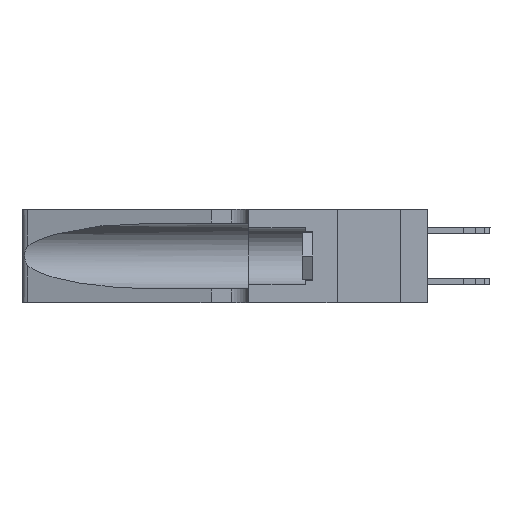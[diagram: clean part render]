
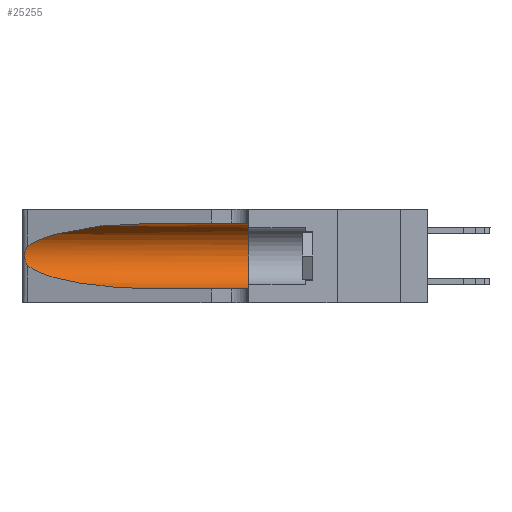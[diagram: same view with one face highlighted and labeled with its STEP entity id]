
A CAD part, left-side view. The second image highlights one B-rep face of the part: STEP entity #25255.
In plain terms, the highlighted cylindrical face has radius 3.308 mm (diameter 6.617 mm), a partial arc.
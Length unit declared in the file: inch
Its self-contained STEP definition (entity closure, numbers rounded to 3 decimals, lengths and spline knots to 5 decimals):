
#773 = DIRECTION ( 'NONE',  ( 0., 0., 1. ) ) ;
#2252 = CARTESIAN_POINT ( 'NONE',  ( 0.1305, 0.72297, 0.31525 ) ) ;
#2629 = LINE ( 'NONE', #6102, #7600 ) ;
#2681 = B_SPLINE_CURVE_WITH_KNOTS ( 'NONE', 3,
 ( #25876, #13319, #20587, #30576, #18399, #15840, #3589, #23060, #10579, #8186, #25547, #28333, #16072, #28000 ),
 .UNSPECIFIED., .F., .F.,
 ( 4, 2, 2, 2, 2, 2, 4 ),
 ( 0., 0.00027, 0.00053, 0.00107, 0.0016, 0.00187, 0.00214 ),
 .UNSPECIFIED. ) ;
#3499 = CARTESIAN_POINT ( 'NONE',  ( 0.1305, 0.35, 0.185 ) ) ;
#3589 = CARTESIAN_POINT ( 'NONE',  ( 0.26075, 1.23896, 0.19203 ) ) ;
#4714 = VERTEX_POINT ( 'NONE', #6596 ) ;
#6102 = CARTESIAN_POINT ( 'NONE',  ( 0.1305, 1.61858, 0.31525 ) ) ;
#6596 = CARTESIAN_POINT ( 'NONE',  ( 0.1305, 0.35, 0.05475 ) ) ;
#7600 = VECTOR ( 'NONE', #18666, 39.37008 ) ;
#7822 = FACE_OUTER_BOUND ( 'NONE', #11271, .T. ) ;
#8050 = CARTESIAN_POINT ( 'NONE',  ( 0.1305, 1.61858, 0.185 ) ) ;
#8186 = CARTESIAN_POINT ( 'NONE',  ( 0.25856, 1.23593, 0.16098 ) ) ;
#8829 = EDGE_CURVE ( 'NONE', #23982, #14994, #9378, .T. ) ;
#8981 = CARTESIAN_POINT ( 'NONE',  ( 0.25487, 1.22718, 0.22369 ) ) ;
#9378 =( BOUNDED_CURVE ( )  B_SPLINE_CURVE ( 3, ( #2252, #29449, #24314, #26797 ),
 .UNSPECIFIED., .F., .T. ) 
 B_SPLINE_CURVE_WITH_KNOTS ( ( 4, 4 ),
 ( 1.5708, 2.84003 ),
 .UNSPECIFIED. ) 
 CURVE ( )  GEOMETRIC_REPRESENTATION_ITEM ( )  RATIONAL_B_SPLINE_CURVE ( ( 1., 0.87, 0.87, 1. ) ) 
 REPRESENTATION_ITEM ( '' )  );
#10579 = CARTESIAN_POINT ( 'NONE',  ( 0.26017, 1.23833, 0.17102 ) ) ;
#10772 =( BOUNDED_CURVE ( )  B_SPLINE_CURVE ( 3, ( #27943, #15438, #13599, #25811 ),
 .UNSPECIFIED., .F., .T. ) 
 B_SPLINE_CURVE_WITH_KNOTS ( ( 4, 4 ),
 ( 3.44316, 4.71239 ),
 .UNSPECIFIED. ) 
 CURVE ( )  GEOMETRIC_REPRESENTATION_ITEM ( )  RATIONAL_B_SPLINE_CURVE ( ( 1., 0.87, 0.87, 1. ) ) 
 REPRESENTATION_ITEM ( '' )  );
#11271 = EDGE_LOOP ( 'NONE', ( #30564, #14636, #17746, #25614, #18194, #31581 ) ) ;
#11343 = LINE ( 'NONE', #31192, #18331 ) ;
#13159 = EDGE_CURVE ( 'NONE', #23982, #17050, #2629, .T. ) ;
#13319 = CARTESIAN_POINT ( 'NONE',  ( 0.25555, 1.22994, 0.2215 ) ) ;
#13599 = CARTESIAN_POINT ( 'NONE',  ( 0.18966, 0.96281, 0.05475 ) ) ;
#13842 = CARTESIAN_POINT ( 'NONE',  ( 0.25487, 1.22718, 0.14631 ) ) ;
#14411 = EDGE_CURVE ( 'NONE', #24363, #4714, #11343, .T. ) ;
#14636 = ORIENTED_EDGE ( 'NONE', *, *, #16585, .T. ) ;
#14994 = VERTEX_POINT ( 'NONE', #8981 ) ;
#15263 = DIRECTION ( 'NONE',  ( 0., 0., -1. ) ) ;
#15438 = CARTESIAN_POINT ( 'NONE',  ( 0.2373, 1.15595, 0.08982 ) ) ;
#15840 = CARTESIAN_POINT ( 'NONE',  ( 0.26018, 1.23835, 0.19895 ) ) ;
#16072 = CARTESIAN_POINT ( 'NONE',  ( 0.25555, 1.22993, 0.14849 ) ) ;
#16462 = DIRECTION ( 'NONE',  ( 0., -1., 0. ) ) ;
#16504 = CIRCLE ( 'NONE', #19438, 0.13025 ) ;
#16585 = EDGE_CURVE ( 'NONE', #14994, #30152, #2681, .T. ) ;
#17050 = VERTEX_POINT ( 'NONE', #23810 ) ;
#17746 = ORIENTED_EDGE ( 'NONE', *, *, #21532, .T. ) ;
#18194 = ORIENTED_EDGE ( 'NONE', *, *, #24728, .F. ) ;
#18331 = VECTOR ( 'NONE', #16462, 39.37008 ) ;
#18399 = CARTESIAN_POINT ( 'NONE',  ( 0.25854, 1.2359, 0.20912 ) ) ;
#18666 = DIRECTION ( 'NONE',  ( 0., -1., 0. ) ) ;
#19438 = AXIS2_PLACEMENT_3D ( 'NONE', #3499, #25339, #773 ) ;
#20450 = DIRECTION ( 'NONE',  ( 0., -1., 0. ) ) ;
#20587 = CARTESIAN_POINT ( 'NONE',  ( 0.25639, 1.23184, 0.21858 ) ) ;
#21532 = EDGE_CURVE ( 'NONE', #30152, #24363, #10772, .T. ) ;
#23060 = CARTESIAN_POINT ( 'NONE',  ( 0.26075, 1.23896, 0.178 ) ) ;
#23810 = CARTESIAN_POINT ( 'NONE',  ( 0.1305, 0.35, 0.31525 ) ) ;
#23982 = VERTEX_POINT ( 'NONE', #26019 ) ;
#24314 = CARTESIAN_POINT ( 'NONE',  ( 0.2373, 1.15595, 0.28018 ) ) ;
#24363 = VERTEX_POINT ( 'NONE', #26675 ) ;
#24728 = EDGE_CURVE ( 'NONE', #17050, #4714, #16504, .T. ) ;
#25255 = ADVANCED_FACE ( 'NONE', ( #7822 ), #27596, .F. ) ;
#25339 = DIRECTION ( 'NONE',  ( 0., 1., 0. ) ) ;
#25547 = CARTESIAN_POINT ( 'NONE',  ( 0.25789, 1.23486, 0.15765 ) ) ;
#25614 = ORIENTED_EDGE ( 'NONE', *, *, #14411, .T. ) ;
#25811 = CARTESIAN_POINT ( 'NONE',  ( 0.1305, 0.72297, 0.05475 ) ) ;
#25876 = CARTESIAN_POINT ( 'NONE',  ( 0.25487, 1.22718, 0.22369 ) ) ;
#26019 = CARTESIAN_POINT ( 'NONE',  ( 0.1305, 0.72297, 0.31525 ) ) ;
#26675 = CARTESIAN_POINT ( 'NONE',  ( 0.1305, 0.72297, 0.05475 ) ) ;
#26797 = CARTESIAN_POINT ( 'NONE',  ( 0.25487, 1.22718, 0.22369 ) ) ;
#27596 = CYLINDRICAL_SURFACE ( 'NONE', #31232, 0.13025 ) ;
#27943 = CARTESIAN_POINT ( 'NONE',  ( 0.25487, 1.22718, 0.14631 ) ) ;
#28000 = CARTESIAN_POINT ( 'NONE',  ( 0.25487, 1.22718, 0.14631 ) ) ;
#28333 = CARTESIAN_POINT ( 'NONE',  ( 0.25639, 1.23186, 0.15144 ) ) ;
#29449 = CARTESIAN_POINT ( 'NONE',  ( 0.18966, 0.96281, 0.31525 ) ) ;
#30152 = VERTEX_POINT ( 'NONE', #13842 ) ;
#30564 = ORIENTED_EDGE ( 'NONE', *, *, #8829, .T. ) ;
#30576 = CARTESIAN_POINT ( 'NONE',  ( 0.25787, 1.23484, 0.2124 ) ) ;
#31192 = CARTESIAN_POINT ( 'NONE',  ( 0.1305, 1.61858, 0.05475 ) ) ;
#31232 = AXIS2_PLACEMENT_3D ( 'NONE', #8050, #20450, #15263 ) ;
#31581 = ORIENTED_EDGE ( 'NONE', *, *, #13159, .F. ) ;
